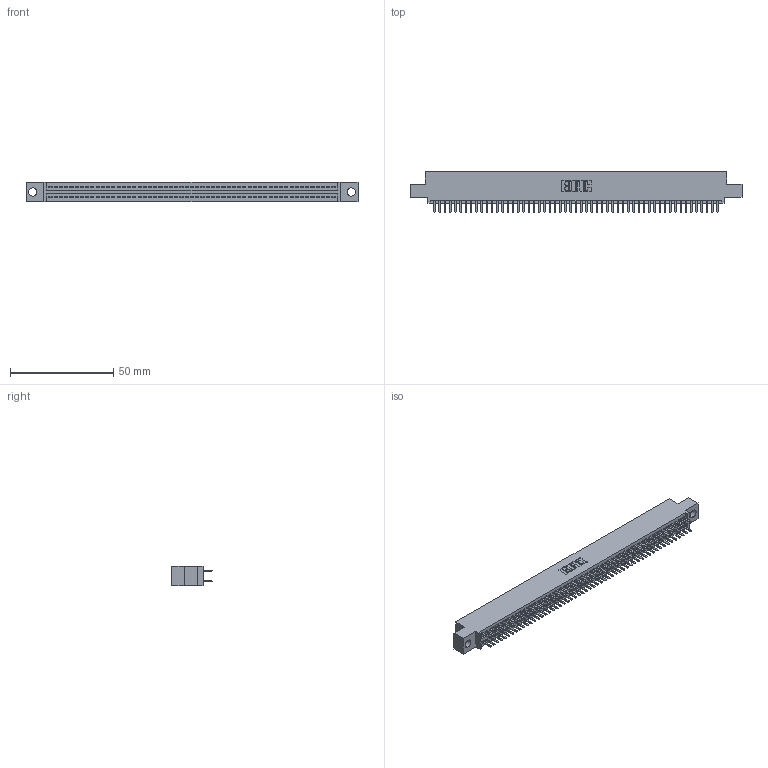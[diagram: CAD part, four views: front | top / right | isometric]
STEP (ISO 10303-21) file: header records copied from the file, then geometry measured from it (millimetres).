
FILE_DESCRIPTION (( 'STEP AP203' ), '1' );
FILE_NAME ('395-110-520-504.STEP', '2021-06-17T17:29:46', ( '' ), ( '' ), 'SwSTEP 2.0', 'SolidWorks 2020', '' );
FILE_SCHEMA (( 'CONFIG_CONTROL_DESIGN' ));
Length unit declared in the file: inch
Products named in the file (3): 345 Part_0.110 Offset - 0.156 Dia-TI; 395-110-520-504; 345-292-001_345-293-120
Assembly tree (111 placements, depth 2):
  395-110-520-504
    345 Part_0.110 Offset - 0.156 Dia-TI
    345-292-001_345-293-120  x110
Bounding box: 160.91 x 19.68 x 9.4 mm (x, y, z)
Volume: 15523.9 mm3; surface area: 23040.2 mm2
Topology: 111 solids, 111 shells, 6084 faces, 17659 edges, 11478 vertices
Faces by surface type: plane 3948, cylinder 2136
Entity records: 42069 total; most frequent: CARTESIAN_POINT 7058, ORIENTED_EDGE 6978, DIRECTION 6193, EDGE_CURVE 3489, VECTOR 3133, LINE 3133, VERTEX_POINT 2322, AXIS2_PLACEMENT_3D 1530
